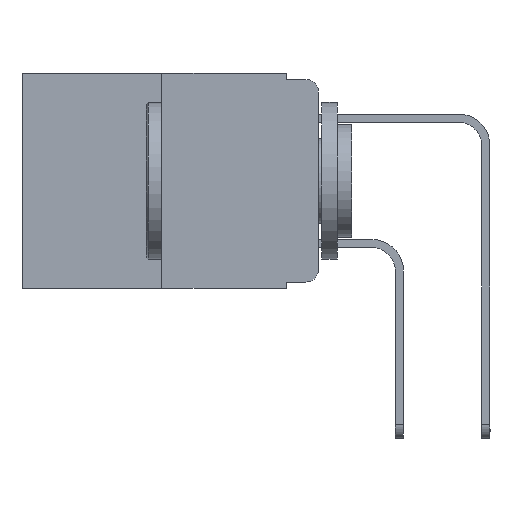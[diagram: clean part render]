
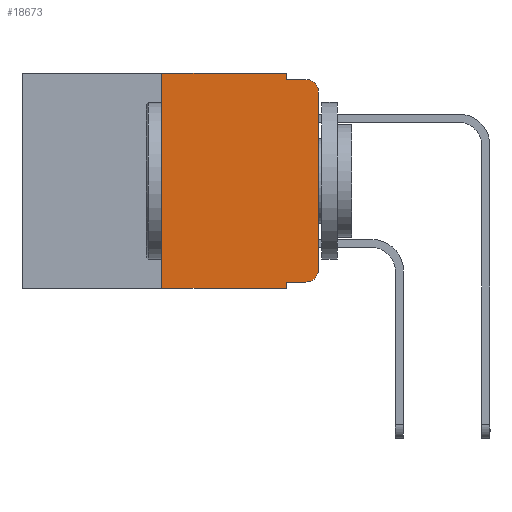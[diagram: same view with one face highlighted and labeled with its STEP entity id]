
A CAD part, left-side view. The second image highlights one B-rep face of the part: STEP entity #18673.
In plain terms, the highlighted planar face has unit normal (-1, 0, 0).
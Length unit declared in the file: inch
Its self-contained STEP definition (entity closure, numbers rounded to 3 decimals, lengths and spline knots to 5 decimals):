
#71 = DIRECTION ( 'NONE',  ( 0., -1., 0. ) ) ;
#121 = VERTEX_POINT ( 'NONE', #494 ) ;
#145 = CARTESIAN_POINT ( 'NONE',  ( 0., 0.25, -0.343 ) ) ;
#468 = VECTOR ( 'NONE', #12434, 39.37008 ) ;
#494 = CARTESIAN_POINT ( 'NONE',  ( 0., 0.051, -0.343 ) ) ;
#509 = DIRECTION ( 'NONE',  ( 0., 0., -1. ) ) ;
#587 = ORIENTED_EDGE ( 'NONE', *, *, #12358, .F. ) ;
#757 = DIRECTION ( 'NONE',  ( -1., 0., 0. ) ) ;
#850 = LINE ( 'NONE', #10642, #8103 ) ;
#974 = LINE ( 'NONE', #3278, #19628 ) ;
#1222 = DIRECTION ( 'NONE',  ( 0., 0., 1. ) ) ;
#1388 = EDGE_CURVE ( 'NONE', #13710, #121, #850, .T. ) ;
#1549 = CIRCLE ( 'NONE', #1942, 0.02 ) ;
#1793 = VERTEX_POINT ( 'NONE', #5056 ) ;
#1942 = AXIS2_PLACEMENT_3D ( 'NONE', #15368, #8692, #12312 ) ;
#2074 = CARTESIAN_POINT ( 'NONE',  ( 0., 0., -0.03 ) ) ;
#2134 = EDGE_LOOP ( 'NONE', ( #3827, #6991, #18102, #14845, #10645, #587, #6348, #3126, #11719, #11805 ) ) ;
#3126 = ORIENTED_EDGE ( 'NONE', *, *, #1388, .F. ) ;
#3278 = CARTESIAN_POINT ( 'NONE',  ( 0., 0.051, -0.01 ) ) ;
#3618 = AXIS2_PLACEMENT_3D ( 'NONE', #19365, #20898, #5975 ) ;
#3827 = ORIENTED_EDGE ( 'NONE', *, *, #11322, .T. ) ;
#3983 = CARTESIAN_POINT ( 'NONE',  ( 0., 0.25, 0. ) ) ;
#4223 = CARTESIAN_POINT ( 'NONE',  ( 0., 0.051, -0.333 ) ) ;
#4448 = LINE ( 'NONE', #3983, #7567 ) ;
#4817 = DIRECTION ( 'NONE',  ( 0., -1., 0. ) ) ;
#5056 = CARTESIAN_POINT ( 'NONE',  ( 0., 0., -0.313 ) ) ;
#5148 = VECTOR ( 'NONE', #20025, 39.37008 ) ;
#5321 = EDGE_CURVE ( 'NONE', #19061, #15353, #974, .T. ) ;
#5900 = LINE ( 'NONE', #8420, #11876 ) ;
#5975 = DIRECTION ( 'NONE',  ( 0., 0., -1. ) ) ;
#5977 = CARTESIAN_POINT ( 'NONE',  ( 0., 0.02, -0.333 ) ) ;
#6348 = ORIENTED_EDGE ( 'NONE', *, *, #20761, .T. ) ;
#6655 = CARTESIAN_POINT ( 'NONE',  ( 0., 0.473, 0. ) ) ;
#6736 = EDGE_CURVE ( 'NONE', #18315, #19061, #13229, .T. ) ;
#6944 = CIRCLE ( 'NONE', #8605, 0.02 ) ;
#6991 = ORIENTED_EDGE ( 'NONE', *, *, #14726, .T. ) ;
#7294 = EDGE_CURVE ( 'NONE', #13710, #11910, #20458, .T. ) ;
#7380 = DIRECTION ( 'NONE',  ( 0., 0., -1. ) ) ;
#7567 = VECTOR ( 'NONE', #12190, 39.37008 ) ;
#8103 = VECTOR ( 'NONE', #7380, 39.37008 ) ;
#8155 = CARTESIAN_POINT ( 'NONE',  ( 0., 0.051, 0. ) ) ;
#8420 = CARTESIAN_POINT ( 'NONE',  ( 0., 0.473, -0.343 ) ) ;
#8605 = AXIS2_PLACEMENT_3D ( 'NONE', #13840, #757, #20474 ) ;
#8692 = DIRECTION ( 'NONE',  ( -1., 0., 0. ) ) ;
#9250 = CARTESIAN_POINT ( 'NONE',  ( 0., 0.051, -0.333 ) ) ;
#9443 = PLANE ( 'NONE',  #3618 ) ;
#9943 = VECTOR ( 'NONE', #1222, 39.37008 ) ;
#10430 = CARTESIAN_POINT ( 'NONE',  ( 0., 0.051, -0.01 ) ) ;
#10642 = CARTESIAN_POINT ( 'NONE',  ( 0., 0.051, 0. ) ) ;
#10645 = ORIENTED_EDGE ( 'NONE', *, *, #15310, .F. ) ;
#11322 = EDGE_CURVE ( 'NONE', #1793, #11663, #13313, .T. ) ;
#11663 = VERTEX_POINT ( 'NONE', #2074 ) ;
#11719 = ORIENTED_EDGE ( 'NONE', *, *, #7294, .T. ) ;
#11805 = ORIENTED_EDGE ( 'NONE', *, *, #15459, .T. ) ;
#11876 = VECTOR ( 'NONE', #71, 39.37008 ) ;
#11910 = VERTEX_POINT ( 'NONE', #5977 ) ;
#12190 = DIRECTION ( 'NONE',  ( 0., 0., 1. ) ) ;
#12312 = DIRECTION ( 'NONE',  ( 0., 0., -1. ) ) ;
#12358 = EDGE_CURVE ( 'NONE', #14074, #16700, #4448, .T. ) ;
#12434 = DIRECTION ( 'NONE',  ( 0., -1., 0. ) ) ;
#13229 = LINE ( 'NONE', #20388, #19455 ) ;
#13313 = LINE ( 'NONE', #21073, #9943 ) ;
#13710 = VERTEX_POINT ( 'NONE', #4223 ) ;
#13731 = CARTESIAN_POINT ( 'NONE',  ( 0., 0.25, 0. ) ) ;
#13840 = CARTESIAN_POINT ( 'NONE',  ( 0., 0.02, -0.313 ) ) ;
#14074 = VERTEX_POINT ( 'NONE', #145 ) ;
#14726 = EDGE_CURVE ( 'NONE', #11663, #15353, #1549, .T. ) ;
#14845 = ORIENTED_EDGE ( 'NONE', *, *, #6736, .F. ) ;
#15139 = CARTESIAN_POINT ( 'NONE',  ( 0., 0.02, -0.01 ) ) ;
#15310 = EDGE_CURVE ( 'NONE', #16700, #18315, #20157, .T. ) ;
#15353 = VERTEX_POINT ( 'NONE', #15139 ) ;
#15368 = CARTESIAN_POINT ( 'NONE',  ( 0., 0.02, -0.03 ) ) ;
#15459 = EDGE_CURVE ( 'NONE', #11910, #1793, #6944, .T. ) ;
#16700 = VERTEX_POINT ( 'NONE', #13731 ) ;
#18102 = ORIENTED_EDGE ( 'NONE', *, *, #5321, .F. ) ;
#18315 = VERTEX_POINT ( 'NONE', #8155 ) ;
#18673 = ADVANCED_FACE ( 'NONE', ( #21100 ), #9443, .F. ) ;
#19061 = VERTEX_POINT ( 'NONE', #10430 ) ;
#19365 = CARTESIAN_POINT ( 'NONE',  ( 0., 0.473, 0. ) ) ;
#19455 = VECTOR ( 'NONE', #509, 39.37008 ) ;
#19628 = VECTOR ( 'NONE', #4817, 39.37008 ) ;
#20025 = DIRECTION ( 'NONE',  ( 0., -1., 0. ) ) ;
#20157 = LINE ( 'NONE', #6655, #5148 ) ;
#20388 = CARTESIAN_POINT ( 'NONE',  ( 0., 0.051, 0. ) ) ;
#20458 = LINE ( 'NONE', #9250, #468 ) ;
#20474 = DIRECTION ( 'NONE',  ( 0., 0., -1. ) ) ;
#20761 = EDGE_CURVE ( 'NONE', #14074, #121, #5900, .T. ) ;
#20898 = DIRECTION ( 'NONE',  ( 1., 0., 0. ) ) ;
#21073 = CARTESIAN_POINT ( 'NONE',  ( 0., 0., 0. ) ) ;
#21100 = FACE_OUTER_BOUND ( 'NONE', #2134, .T. ) ;
